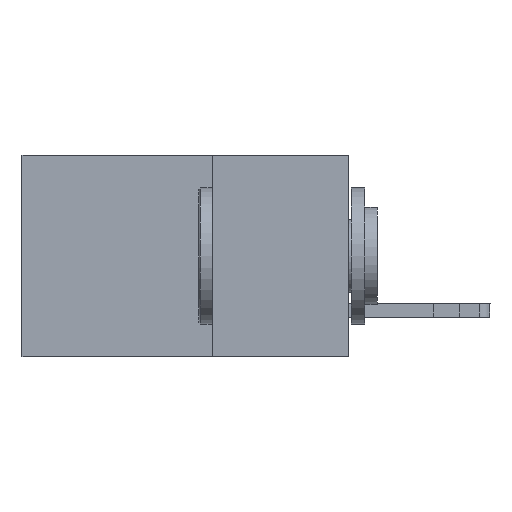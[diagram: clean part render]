
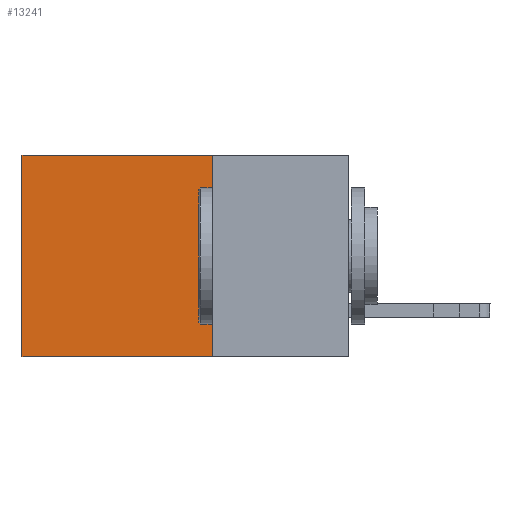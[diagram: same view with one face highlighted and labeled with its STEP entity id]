
A CAD part, left-side view. The second image highlights one B-rep face of the part: STEP entity #13241.
In plain terms, the highlighted planar face has unit normal (-1, 0, 0).
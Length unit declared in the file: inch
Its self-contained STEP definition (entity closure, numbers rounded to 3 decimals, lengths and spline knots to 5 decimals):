
#820 = CARTESIAN_POINT ( 'NONE',  ( 0.2615, 0.25, -0.37 ) ) ;
#1182 = VECTOR ( 'NONE', #1737, 39.37008 ) ;
#1190 = VERTEX_POINT ( 'NONE', #820 ) ;
#1411 = DIRECTION ( 'NONE',  ( 0., 0., -1. ) ) ;
#1622 = CARTESIAN_POINT ( 'NONE',  ( 0.2615, 0.25, -0.37 ) ) ;
#1737 = DIRECTION ( 'NONE',  ( 0., 1., 0. ) ) ;
#2469 = CARTESIAN_POINT ( 'NONE',  ( 0.2615, 0.6, 0. ) ) ;
#2520 = ORIENTED_EDGE ( 'NONE', *, *, #9300, .T. ) ;
#2605 = VERTEX_POINT ( 'NONE', #2469 ) ;
#2646 = AXIS2_PLACEMENT_3D ( 'NONE', #7839, #4286, #12513 ) ;
#3091 = PLANE ( 'NONE',  #2646 ) ;
#4286 = DIRECTION ( 'NONE',  ( 1., 0., 0. ) ) ;
#5071 = LINE ( 'NONE', #12315, #1182 ) ;
#5224 = CARTESIAN_POINT ( 'NONE',  ( 0.2615, 0.25, 0. ) ) ;
#5546 = CARTESIAN_POINT ( 'NONE',  ( 0.2615, 0.6, -0.37 ) ) ;
#5815 = FACE_OUTER_BOUND ( 'NONE', #10105, .T. ) ;
#6421 = DIRECTION ( 'NONE',  ( 0., 1., 0. ) ) ;
#6457 = LINE ( 'NONE', #5224, #12332 ) ;
#7336 = EDGE_CURVE ( 'NONE', #13565, #1190, #10074, .T. ) ;
#7417 = VECTOR ( 'NONE', #11365, 39.37008 ) ;
#7468 = EDGE_CURVE ( 'NONE', #1190, #7602, #5071, .T. ) ;
#7602 = VERTEX_POINT ( 'NONE', #5546 ) ;
#7839 = CARTESIAN_POINT ( 'NONE',  ( 0.2615, 0.25, -0.37 ) ) ;
#9300 = EDGE_CURVE ( 'NONE', #13565, #2605, #6457, .T. ) ;
#9333 = VECTOR ( 'NONE', #1411, 39.37008 ) ;
#9431 = EDGE_CURVE ( 'NONE', #2605, #7602, #10886, .T. ) ;
#10074 = LINE ( 'NONE', #1622, #9333 ) ;
#10105 = EDGE_LOOP ( 'NONE', ( #12115, #11438, #13193, #2520 ) ) ;
#10886 = LINE ( 'NONE', #13632, #7417 ) ;
#11365 = DIRECTION ( 'NONE',  ( 0., 0., -1. ) ) ;
#11438 = ORIENTED_EDGE ( 'NONE', *, *, #7468, .F. ) ;
#12115 = ORIENTED_EDGE ( 'NONE', *, *, #9431, .T. ) ;
#12315 = CARTESIAN_POINT ( 'NONE',  ( 0.2615, 0.25, -0.37 ) ) ;
#12332 = VECTOR ( 'NONE', #6421, 39.37008 ) ;
#12513 = DIRECTION ( 'NONE',  ( 0., 0., -1. ) ) ;
#13193 = ORIENTED_EDGE ( 'NONE', *, *, #7336, .F. ) ;
#13241 = ADVANCED_FACE ( 'NONE', ( #5815 ), #3091, .F. ) ;
#13565 = VERTEX_POINT ( 'NONE', #15167 ) ;
#13632 = CARTESIAN_POINT ( 'NONE',  ( 0.2615, 0.6, -0.37 ) ) ;
#15167 = CARTESIAN_POINT ( 'NONE',  ( 0.2615, 0.25, 0. ) ) ;
